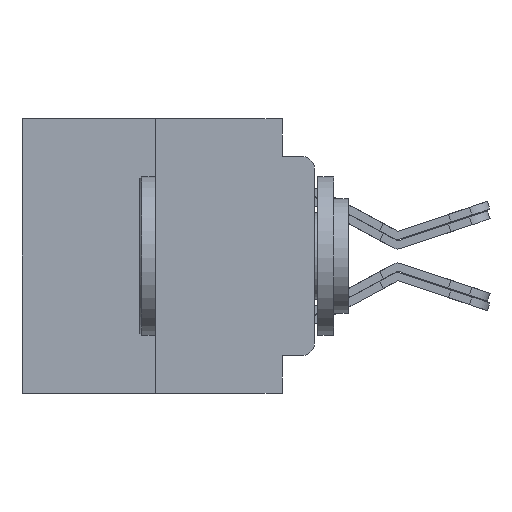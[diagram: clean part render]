
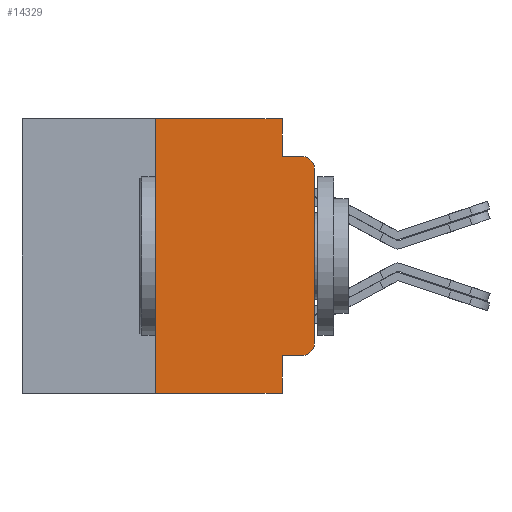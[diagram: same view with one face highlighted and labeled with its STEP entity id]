
A CAD part, left-side view. The second image highlights one B-rep face of the part: STEP entity #14329.
In plain terms, the highlighted planar face has unit normal (-1, 0, 0).
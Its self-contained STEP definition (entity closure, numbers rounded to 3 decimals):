
#5 = VERTEX_POINT ( 'NONE', #17736 ) ;
#58 = VERTEX_POINT ( 'NONE', #18451 ) ;
#773 = VECTOR ( 'NONE', #11670, 1000. ) ;
#839 = AXIS2_PLACEMENT_3D ( 'NONE', #20362, #20569, #4253 ) ;
#1120 = VERTEX_POINT ( 'NONE', #28828 ) ;
#1719 = CARTESIAN_POINT ( 'NONE',  ( -75.603, 0.508, -3.467 ) ) ;
#1826 = CARTESIAN_POINT ( 'NONE',  ( -75.603, 11.684, 5.486 ) ) ;
#1939 = ORIENTED_EDGE ( 'NONE', *, *, #14403, .T. ) ;
#2828 = DIRECTION ( 'NONE',  ( 0., 0., -1. ) ) ;
#2942 = EDGE_CURVE ( 'NONE', #1120, #5, #19899, .T. ) ;
#3256 = VERTEX_POINT ( 'NONE', #12705 ) ;
#4253 = DIRECTION ( 'NONE',  ( 0., 0., -1. ) ) ;
#4262 = DIRECTION ( 'NONE',  ( 0., -1., 0. ) ) ;
#4820 = CARTESIAN_POINT ( 'NONE',  ( -75.603, 1.295, 3.975 ) ) ;
#4977 = AXIS2_PLACEMENT_3D ( 'NONE', #1719, #22419, #8494 ) ;
#5323 = LINE ( 'NONE', #7544, #20999 ) ;
#6044 = VERTEX_POINT ( 'NONE', #22038 ) ;
#6409 = CARTESIAN_POINT ( 'NONE',  ( -75.603, 1.295, -3.975 ) ) ;
#6515 = PLANE ( 'NONE',  #839 ) ;
#6966 = CARTESIAN_POINT ( 'NONE',  ( -75.603, 0.508, -3.975 ) ) ;
#7404 = DIRECTION ( 'NONE',  ( -1., 0., 0. ) ) ;
#7469 = CIRCLE ( 'NONE', #4977, 0.508 ) ;
#7544 = CARTESIAN_POINT ( 'NONE',  ( -75.603, 1.295, 0. ) ) ;
#8494 = DIRECTION ( 'NONE',  ( 0., 0., -1. ) ) ;
#8830 = ORIENTED_EDGE ( 'NONE', *, *, #10479, .F. ) ;
#9730 = FACE_OUTER_BOUND ( 'NONE', #20022, .T. ) ;
#9870 = CARTESIAN_POINT ( 'NONE',  ( -75.603, 1.295, 3.975 ) ) ;
#10082 = VECTOR ( 'NONE', #29813, 1000. ) ;
#10479 = EDGE_CURVE ( 'NONE', #3256, #1120, #14738, .T. ) ;
#10536 = ORIENTED_EDGE ( 'NONE', *, *, #20940, .F. ) ;
#10576 = EDGE_CURVE ( 'NONE', #28302, #11243, #27457, .T. ) ;
#11243 = VERTEX_POINT ( 'NONE', #19254 ) ;
#11670 = DIRECTION ( 'NONE',  ( 0., 0., 1. ) ) ;
#11976 = ORIENTED_EDGE ( 'NONE', *, *, #26378, .T. ) ;
#12056 = VECTOR ( 'NONE', #21318, 1000. ) ;
#12373 = VECTOR ( 'NONE', #17744, 1000. ) ;
#12599 = EDGE_CURVE ( 'NONE', #6044, #28302, #17822, .T. ) ;
#12705 = CARTESIAN_POINT ( 'NONE',  ( -75.603, 6.35, -5.486 ) ) ;
#12954 = ORIENTED_EDGE ( 'NONE', *, *, #24807, .F. ) ;
#14329 = ADVANCED_FACE ( 'NONE', ( #9730 ), #6515, .F. ) ;
#14400 = DIRECTION ( 'NONE',  ( 0., 0., -1. ) ) ;
#14403 = EDGE_CURVE ( 'NONE', #58, #25311, #16979, .T. ) ;
#14738 = LINE ( 'NONE', #25513, #773 ) ;
#15166 = ORIENTED_EDGE ( 'NONE', *, *, #21301, .F. ) ;
#16161 = LINE ( 'NONE', #17468, #24187 ) ;
#16979 = LINE ( 'NONE', #6409, #10082 ) ;
#17133 = LINE ( 'NONE', #4820, #12056 ) ;
#17468 = CARTESIAN_POINT ( 'NONE',  ( -75.603, 11.684, -5.486 ) ) ;
#17736 = CARTESIAN_POINT ( 'NONE',  ( -75.603, 1.295, 5.486 ) ) ;
#17744 = DIRECTION ( 'NONE',  ( 0., 0., 1. ) ) ;
#17822 = LINE ( 'NONE', #22461, #12373 ) ;
#18012 = DIRECTION ( 'NONE',  ( 0., 0., -1. ) ) ;
#18076 = VECTOR ( 'NONE', #4262, 1000. ) ;
#18451 = CARTESIAN_POINT ( 'NONE',  ( -75.603, 1.295, -3.975 ) ) ;
#18561 = ORIENTED_EDGE ( 'NONE', *, *, #12599, .T. ) ;
#18796 = CARTESIAN_POINT ( 'NONE',  ( -75.603, 0.508, 3.467 ) ) ;
#19254 = CARTESIAN_POINT ( 'NONE',  ( -75.603, 0.508, 3.975 ) ) ;
#19886 = VERTEX_POINT ( 'NONE', #9870 ) ;
#19899 = LINE ( 'NONE', #1826, #18076 ) ;
#20022 = EDGE_LOOP ( 'NONE', ( #1939, #22144, #18561, #30050, #10536, #12954, #26469, #8830, #11976, #15166 ) ) ;
#20026 = DIRECTION ( 'NONE',  ( 0., -1., 0. ) ) ;
#20362 = CARTESIAN_POINT ( 'NONE',  ( -75.603, 11.684, 5.486 ) ) ;
#20569 = DIRECTION ( 'NONE',  ( 1., 0., 0. ) ) ;
#20940 = EDGE_CURVE ( 'NONE', #19886, #11243, #17133, .T. ) ;
#20999 = VECTOR ( 'NONE', #2828, 1000. ) ;
#21001 = VERTEX_POINT ( 'NONE', #26610 ) ;
#21301 = EDGE_CURVE ( 'NONE', #58, #21001, #28064, .T. ) ;
#21318 = DIRECTION ( 'NONE',  ( 0., -1., 0. ) ) ;
#22038 = CARTESIAN_POINT ( 'NONE',  ( -75.603, 0., -3.467 ) ) ;
#22144 = ORIENTED_EDGE ( 'NONE', *, *, #25717, .T. ) ;
#22419 = DIRECTION ( 'NONE',  ( -1., 0., 0. ) ) ;
#22461 = CARTESIAN_POINT ( 'NONE',  ( -75.603, 0., 5.486 ) ) ;
#24187 = VECTOR ( 'NONE', #20026, 1000. ) ;
#24786 = AXIS2_PLACEMENT_3D ( 'NONE', #18796, #7404, #14400 ) ;
#24807 = EDGE_CURVE ( 'NONE', #5, #19886, #5323, .T. ) ;
#25311 = VERTEX_POINT ( 'NONE', #6966 ) ;
#25493 = VECTOR ( 'NONE', #18012, 1000. ) ;
#25513 = CARTESIAN_POINT ( 'NONE',  ( -75.603, 6.35, -5.486 ) ) ;
#25717 = EDGE_CURVE ( 'NONE', #25311, #6044, #7469, .T. ) ;
#26378 = EDGE_CURVE ( 'NONE', #3256, #21001, #16161, .T. ) ;
#26469 = ORIENTED_EDGE ( 'NONE', *, *, #2942, .F. ) ;
#26610 = CARTESIAN_POINT ( 'NONE',  ( -75.603, 1.295, -5.486 ) ) ;
#27457 = CIRCLE ( 'NONE', #24786, 0.508 ) ;
#28064 = LINE ( 'NONE', #29422, #25493 ) ;
#28302 = VERTEX_POINT ( 'NONE', #29650 ) ;
#28828 = CARTESIAN_POINT ( 'NONE',  ( -75.603, 6.35, 5.486 ) ) ;
#29422 = CARTESIAN_POINT ( 'NONE',  ( -75.603, 1.295, 0. ) ) ;
#29650 = CARTESIAN_POINT ( 'NONE',  ( -75.603, 0., 3.467 ) ) ;
#29813 = DIRECTION ( 'NONE',  ( 0., -1., 0. ) ) ;
#30050 = ORIENTED_EDGE ( 'NONE', *, *, #10576, .T. ) ;
